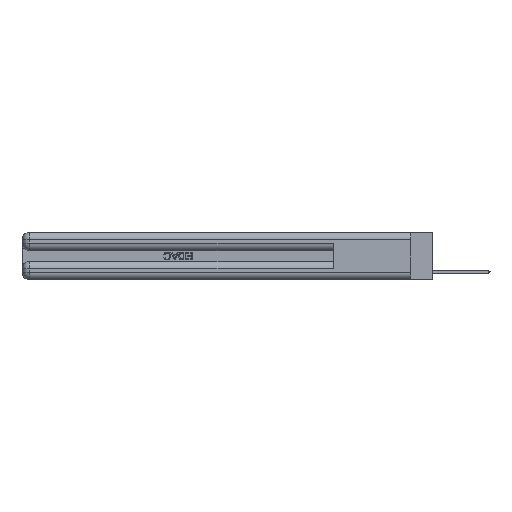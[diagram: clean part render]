
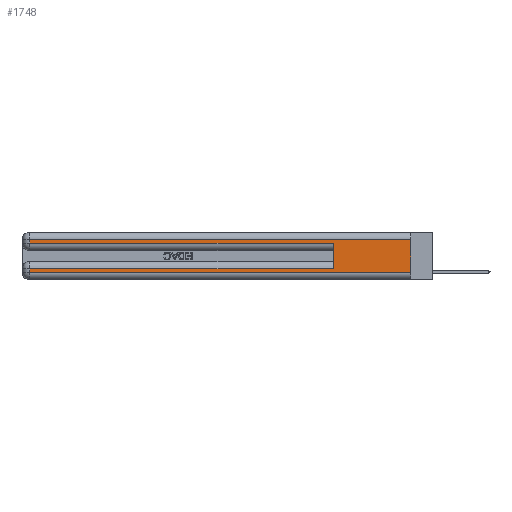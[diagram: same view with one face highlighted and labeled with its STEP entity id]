
A CAD part, left-side view. The second image highlights one B-rep face of the part: STEP entity #1748.
In plain terms, the highlighted planar face has unit normal (-1, 0, 0).
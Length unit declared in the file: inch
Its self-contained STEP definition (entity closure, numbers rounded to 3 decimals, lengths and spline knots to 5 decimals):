
#445 = VERTEX_POINT ( 'NONE', #16014 ) ;
#518 = CARTESIAN_POINT ( 'NONE',  ( 0., 0., 0.37 ) ) ;
#988 = CARTESIAN_POINT ( 'NONE',  ( 0., 0.6, 0.285 ) ) ;
#1483 = EDGE_CURVE ( 'NONE', #18421, #25561, #24608, .T. ) ;
#1748 = ADVANCED_FACE ( 'NONE', ( #25000 ), #2845, .F. ) ;
#2168 = ORIENTED_EDGE ( 'NONE', *, *, #32354, .T. ) ;
#2373 = CARTESIAN_POINT ( 'NONE',  ( 0., 0., 0.085 ) ) ;
#2845 = PLANE ( 'NONE',  #5197 ) ;
#4421 = VECTOR ( 'NONE', #8719, 39.37008 ) ;
#5171 = CARTESIAN_POINT ( 'NONE',  ( 0., 0., 0.285 ) ) ;
#5197 = AXIS2_PLACEMENT_3D ( 'NONE', #518, #5309, #25662 ) ;
#5309 = DIRECTION ( 'NONE',  ( 1., 0., 0. ) ) ;
#5424 = DIRECTION ( 'NONE',  ( 0., 0., 1. ) ) ;
#6433 = ORIENTED_EDGE ( 'NONE', *, *, #9889, .T. ) ;
#7993 = CARTESIAN_POINT ( 'NONE',  ( 0., 2.94, 0.285 ) ) ;
#8563 = DIRECTION ( 'NONE',  ( 0., 0., -1. ) ) ;
#8719 = DIRECTION ( 'NONE',  ( 0., 1., 0. ) ) ;
#9746 = CARTESIAN_POINT ( 'NONE',  ( 0., 0., 0.31 ) ) ;
#9889 = EDGE_CURVE ( 'NONE', #445, #27059, #27628, .T. ) ;
#10853 = CARTESIAN_POINT ( 'NONE',  ( 0., 2.94, 0.085 ) ) ;
#11019 = CARTESIAN_POINT ( 'NONE',  ( 0., 2.94, 0.37 ) ) ;
#11988 = VECTOR ( 'NONE', #29157, 39.37008 ) ;
#12020 = EDGE_LOOP ( 'NONE', ( #28454, #16663, #6433, #22058, #16219, #13015, #12971, #2168 ) ) ;
#12318 = VECTOR ( 'NONE', #12372, 39.37008 ) ;
#12372 = DIRECTION ( 'NONE',  ( 0., 1., 0. ) ) ;
#12971 = ORIENTED_EDGE ( 'NONE', *, *, #14600, .T. ) ;
#13015 = ORIENTED_EDGE ( 'NONE', *, *, #18669, .T. ) ;
#13434 = EDGE_CURVE ( 'NONE', #18421, #445, #22658, .T. ) ;
#14600 = EDGE_CURVE ( 'NONE', #30072, #23353, #19473, .T. ) ;
#14900 = CARTESIAN_POINT ( 'NONE',  ( 0., 0., 0.31 ) ) ;
#15248 = LINE ( 'NONE', #19630, #32254 ) ;
#16014 = CARTESIAN_POINT ( 'NONE',  ( 0., 2.94, 0.31 ) ) ;
#16219 = ORIENTED_EDGE ( 'NONE', *, *, #29897, .F. ) ;
#16663 = ORIENTED_EDGE ( 'NONE', *, *, #13434, .T. ) ;
#16964 = VECTOR ( 'NONE', #8563, 39.37008 ) ;
#18246 = LINE ( 'NONE', #23326, #32487 ) ;
#18421 = VERTEX_POINT ( 'NONE', #9746 ) ;
#18669 = EDGE_CURVE ( 'NONE', #29490, #30072, #20654, .T. ) ;
#19304 = DIRECTION ( 'NONE',  ( 0., 0., -1. ) ) ;
#19473 = LINE ( 'NONE', #27139, #31722 ) ;
#19613 = LINE ( 'NONE', #5171, #27119 ) ;
#19630 = CARTESIAN_POINT ( 'NONE',  ( 0., 0., 0.06 ) ) ;
#20486 = DIRECTION ( 'NONE',  ( 0., -1., 0. ) ) ;
#20654 = LINE ( 'NONE', #2373, #12318 ) ;
#22042 = VERTEX_POINT ( 'NONE', #988 ) ;
#22058 = ORIENTED_EDGE ( 'NONE', *, *, #27578, .T. ) ;
#22658 = LINE ( 'NONE', #14900, #4421 ) ;
#23326 = CARTESIAN_POINT ( 'NONE',  ( 0., 0.6, 0.145 ) ) ;
#23353 = VERTEX_POINT ( 'NONE', #31922 ) ;
#23799 = CARTESIAN_POINT ( 'NONE',  ( 0., 0., 0.37 ) ) ;
#24608 = LINE ( 'NONE', #23799, #11988 ) ;
#25000 = FACE_OUTER_BOUND ( 'NONE', #12020, .T. ) ;
#25561 = VERTEX_POINT ( 'NONE', #32656 ) ;
#25662 = DIRECTION ( 'NONE',  ( 0., 0., -1. ) ) ;
#27059 = VERTEX_POINT ( 'NONE', #7993 ) ;
#27119 = VECTOR ( 'NONE', #20486, 39.37008 ) ;
#27139 = CARTESIAN_POINT ( 'NONE',  ( 0., 2.94, 0.37 ) ) ;
#27578 = EDGE_CURVE ( 'NONE', #27059, #22042, #19613, .T. ) ;
#27628 = LINE ( 'NONE', #11019, #16964 ) ;
#28454 = ORIENTED_EDGE ( 'NONE', *, *, #1483, .F. ) ;
#29157 = DIRECTION ( 'NONE',  ( 0., 0., -1. ) ) ;
#29490 = VERTEX_POINT ( 'NONE', #30575 ) ;
#29897 = EDGE_CURVE ( 'NONE', #29490, #22042, #18246, .T. ) ;
#30072 = VERTEX_POINT ( 'NONE', #10853 ) ;
#30575 = CARTESIAN_POINT ( 'NONE',  ( 0., 0.6, 0.085 ) ) ;
#31722 = VECTOR ( 'NONE', #19304, 39.37008 ) ;
#31922 = CARTESIAN_POINT ( 'NONE',  ( 0., 2.94, 0.06 ) ) ;
#32021 = DIRECTION ( 'NONE',  ( 0., -1., 0. ) ) ;
#32254 = VECTOR ( 'NONE', #32021, 39.37008 ) ;
#32354 = EDGE_CURVE ( 'NONE', #23353, #25561, #15248, .T. ) ;
#32487 = VECTOR ( 'NONE', #5424, 39.37008 ) ;
#32656 = CARTESIAN_POINT ( 'NONE',  ( 0., 0., 0.06 ) ) ;
